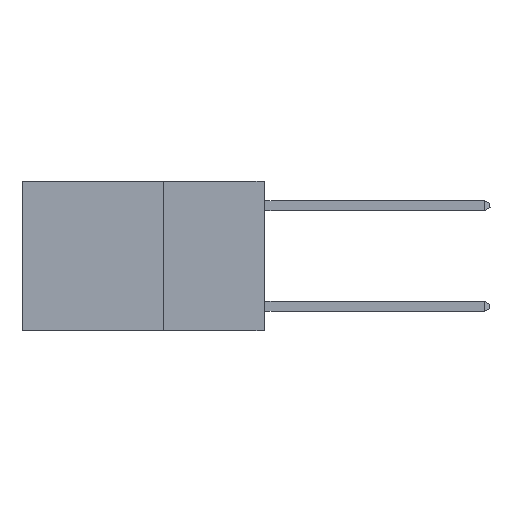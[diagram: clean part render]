
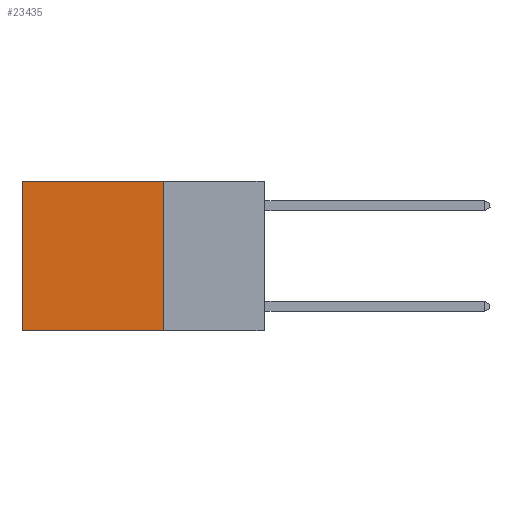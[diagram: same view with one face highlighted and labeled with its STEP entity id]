
A CAD part, left-side view. The second image highlights one B-rep face of the part: STEP entity #23435.
In plain terms, the highlighted planar face has unit normal (-1, 0, 0).
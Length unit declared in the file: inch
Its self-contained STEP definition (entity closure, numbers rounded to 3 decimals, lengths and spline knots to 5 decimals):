
#3978 = ORIENTED_EDGE ( 'NONE', *, *, #28097, .F. ) ;
#4190 = VECTOR ( 'NONE', #22496, 39.37008 ) ;
#5572 = CARTESIAN_POINT ( 'NONE',  ( 0.2625, 0.25, 0. ) ) ;
#7668 = EDGE_LOOP ( 'NONE', ( #12848, #3978, #21973, #17986 ) ) ;
#7704 = DIRECTION ( 'NONE',  ( 0., 1., 0. ) ) ;
#8390 = VERTEX_POINT ( 'NONE', #28003 ) ;
#8441 = VECTOR ( 'NONE', #27686, 39.37008 ) ;
#8838 = VECTOR ( 'NONE', #14619, 39.37008 ) ;
#9055 = VERTEX_POINT ( 'NONE', #10889 ) ;
#9564 = CARTESIAN_POINT ( 'NONE',  ( 0.2625, 0.25, -0.37 ) ) ;
#10889 = CARTESIAN_POINT ( 'NONE',  ( 0.2625, 0.6, 0. ) ) ;
#11166 = VERTEX_POINT ( 'NONE', #5572 ) ;
#12109 = LINE ( 'NONE', #9564, #19355 ) ;
#12724 = EDGE_CURVE ( 'NONE', #11166, #9055, #20207, .T. ) ;
#12848 = ORIENTED_EDGE ( 'NONE', *, *, #18854, .T. ) ;
#13828 = CARTESIAN_POINT ( 'NONE',  ( 0.2625, 0.25, 0. ) ) ;
#13924 = DIRECTION ( 'NONE',  ( 0., 0., -1. ) ) ;
#14619 = DIRECTION ( 'NONE',  ( 0., 0., -1. ) ) ;
#17027 = EDGE_CURVE ( 'NONE', #11166, #20290, #23013, .T. ) ;
#17986 = ORIENTED_EDGE ( 'NONE', *, *, #12724, .T. ) ;
#18197 = CARTESIAN_POINT ( 'NONE',  ( 0.2625, 0.25, -0.37 ) ) ;
#18699 = LINE ( 'NONE', #25538, #8441 ) ;
#18854 = EDGE_CURVE ( 'NONE', #9055, #8390, #18699, .T. ) ;
#19355 = VECTOR ( 'NONE', #7704, 39.37008 ) ;
#20207 = LINE ( 'NONE', #13828, #4190 ) ;
#20290 = VERTEX_POINT ( 'NONE', #18197 ) ;
#20455 = CARTESIAN_POINT ( 'NONE',  ( 0.2625, 0.25, 0. ) ) ;
#21973 = ORIENTED_EDGE ( 'NONE', *, *, #17027, .F. ) ;
#22496 = DIRECTION ( 'NONE',  ( 0., 1., 0. ) ) ;
#23013 = LINE ( 'NONE', #25445, #8838 ) ;
#23092 = AXIS2_PLACEMENT_3D ( 'NONE', #20455, #26871, #13924 ) ;
#23435 = ADVANCED_FACE ( 'NONE', ( #26726 ), #24288, .F. ) ;
#24288 = PLANE ( 'NONE',  #23092 ) ;
#25445 = CARTESIAN_POINT ( 'NONE',  ( 0.2625, 0.25, 0. ) ) ;
#25538 = CARTESIAN_POINT ( 'NONE',  ( 0.2625, 0.6, 0. ) ) ;
#26726 = FACE_OUTER_BOUND ( 'NONE', #7668, .T. ) ;
#26871 = DIRECTION ( 'NONE',  ( 1., 0., 0. ) ) ;
#27686 = DIRECTION ( 'NONE',  ( 0., 0., -1. ) ) ;
#28003 = CARTESIAN_POINT ( 'NONE',  ( 0.2625, 0.6, -0.37 ) ) ;
#28097 = EDGE_CURVE ( 'NONE', #20290, #8390, #12109, .T. ) ;
